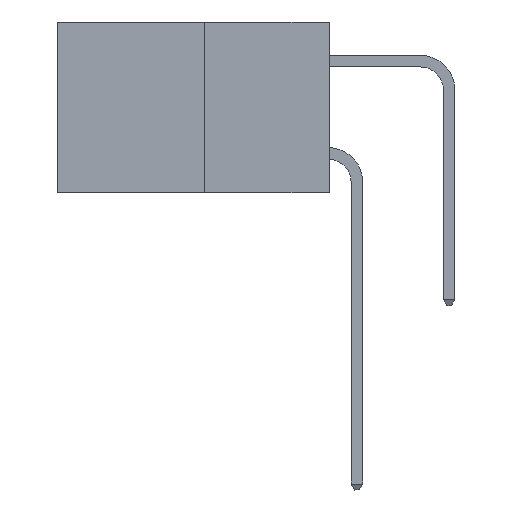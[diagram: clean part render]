
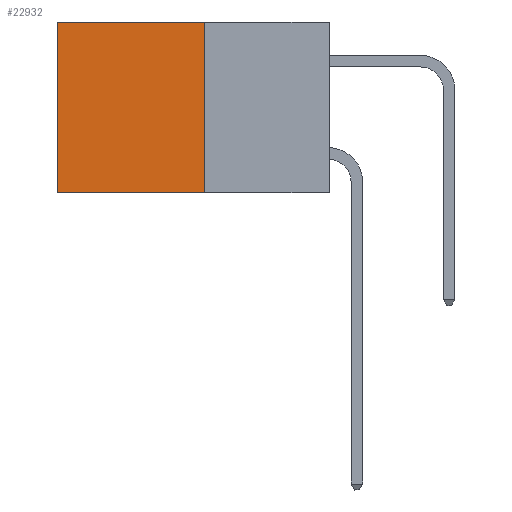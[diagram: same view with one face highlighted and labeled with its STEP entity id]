
A CAD part, left-side view. The second image highlights one B-rep face of the part: STEP entity #22932.
In plain terms, the highlighted planar face has unit normal (-1, 0, 0).
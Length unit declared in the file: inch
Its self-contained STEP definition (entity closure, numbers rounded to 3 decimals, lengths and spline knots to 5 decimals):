
#202 = EDGE_CURVE ( 'NONE', #7058, #8088, #6673, .T. ) ;
#451 = CARTESIAN_POINT ( 'NONE',  ( 0.277, 0.59, -0.37 ) ) ;
#458 = LINE ( 'NONE', #975, #23510 ) ;
#819 = DIRECTION ( 'NONE',  ( 0., 0., -1. ) ) ;
#975 = CARTESIAN_POINT ( 'NONE',  ( 0.277, 0.27, -0.37 ) ) ;
#1286 = VECTOR ( 'NONE', #819, 39.37008 ) ;
#3421 = DIRECTION ( 'NONE',  ( 0., 0., -1. ) ) ;
#3834 = CARTESIAN_POINT ( 'NONE',  ( 0.277, 0.27, -0.37 ) ) ;
#4003 = ORIENTED_EDGE ( 'NONE', *, *, #6393, .T. ) ;
#4650 = VERTEX_POINT ( 'NONE', #5409 ) ;
#4940 = AXIS2_PLACEMENT_3D ( 'NONE', #23425, #14357, #3421 ) ;
#5215 = CARTESIAN_POINT ( 'NONE',  ( 0.277, 0.59, -0.37 ) ) ;
#5409 = CARTESIAN_POINT ( 'NONE',  ( 0.277, 0.59, 0. ) ) ;
#5451 = ORIENTED_EDGE ( 'NONE', *, *, #5773, .F. ) ;
#5773 = EDGE_CURVE ( 'NONE', #8088, #22169, #458, .T. ) ;
#6393 = EDGE_CURVE ( 'NONE', #7058, #4650, #18920, .T. ) ;
#6673 = LINE ( 'NONE', #17579, #1286 ) ;
#7050 = CARTESIAN_POINT ( 'NONE',  ( 0.277, 0.27, 0. ) ) ;
#7058 = VERTEX_POINT ( 'NONE', #7050 ) ;
#7357 = CARTESIAN_POINT ( 'NONE',  ( 0.277, 0.27, 0. ) ) ;
#8088 = VERTEX_POINT ( 'NONE', #3834 ) ;
#8730 = ORIENTED_EDGE ( 'NONE', *, *, #9559, .T. ) ;
#9559 = EDGE_CURVE ( 'NONE', #4650, #22169, #19084, .T. ) ;
#11110 = VECTOR ( 'NONE', #18733, 39.37008 ) ;
#12277 = EDGE_LOOP ( 'NONE', ( #8730, #5451, #18867, #4003 ) ) ;
#12542 = PLANE ( 'NONE',  #4940 ) ;
#13292 = DIRECTION ( 'NONE',  ( 0., 1., 0. ) ) ;
#13716 = DIRECTION ( 'NONE',  ( 0., 1., 0. ) ) ;
#14084 = VECTOR ( 'NONE', #13292, 39.37008 ) ;
#14357 = DIRECTION ( 'NONE',  ( 1., 0., 0. ) ) ;
#17579 = CARTESIAN_POINT ( 'NONE',  ( 0.277, 0.27, -0.37 ) ) ;
#17610 = FACE_OUTER_BOUND ( 'NONE', #12277, .T. ) ;
#18733 = DIRECTION ( 'NONE',  ( 0., 0., -1. ) ) ;
#18867 = ORIENTED_EDGE ( 'NONE', *, *, #202, .F. ) ;
#18920 = LINE ( 'NONE', #7357, #14084 ) ;
#19084 = LINE ( 'NONE', #451, #11110 ) ;
#22169 = VERTEX_POINT ( 'NONE', #5215 ) ;
#22932 = ADVANCED_FACE ( 'NONE', ( #17610 ), #12542, .F. ) ;
#23425 = CARTESIAN_POINT ( 'NONE',  ( 0.277, 0.27, -0.37 ) ) ;
#23510 = VECTOR ( 'NONE', #13716, 39.37008 ) ;
